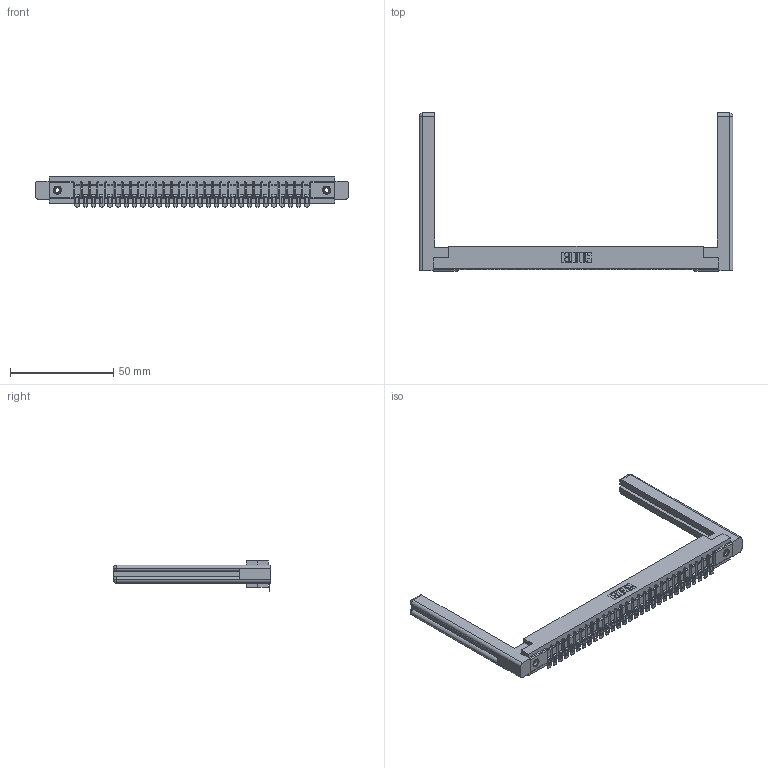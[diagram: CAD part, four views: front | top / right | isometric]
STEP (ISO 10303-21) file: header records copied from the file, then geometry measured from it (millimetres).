
FILE_DESCRIPTION (( 'STEP AP203' ), '1' );
FILE_NAME ('307-029-554-158.STEP', '2019-09-05T03:52:12', ( '' ), ( '' ), 'SwSTEP 2.0', 'SolidWorks 2016', '' );
FILE_SCHEMA (( 'CONFIG_CONTROL_DESIGN' ));
Length unit declared in the file: inch
Products named in the file (5): 307-220-058; 307-029-554-158; 307-290-002_554; 345-250-001_345-250-001-102; 307 Part_.156 Dia Mounting Holes
Assembly tree (34 placements, depth 2):
  307-029-554-158
    307 Part_.156 Dia Mounting Holes
    307-290-002_554  x29
    307-220-058  x2
    345-250-001_345-250-001-102  x2
Bounding box: 151.54 x 76.33 x 14.52 mm (x, y, z)
Volume: 23250.1 mm3; surface area: 24939.9 mm2
Topology: 34 solids, 34 shells, 2639 faces, 8014 edges, 5248 vertices
Faces by surface type: plane 1488, cylinder 1067, sphere 60, torus 12, cone 12
Entity records: 30062 total; most frequent: CARTESIAN_POINT 5077, ORIENTED_EDGE 5006, DIRECTION 4905, EDGE_CURVE 2503, VECTOR 1901, LINE 1901, VERTEX_POINT 1620, AXIS2_PLACEMENT_3D 1502
